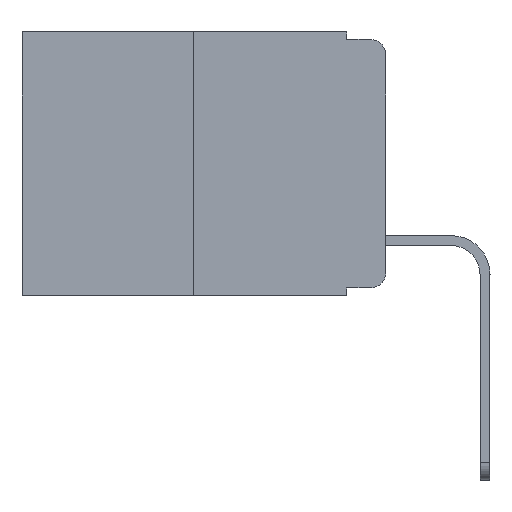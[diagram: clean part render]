
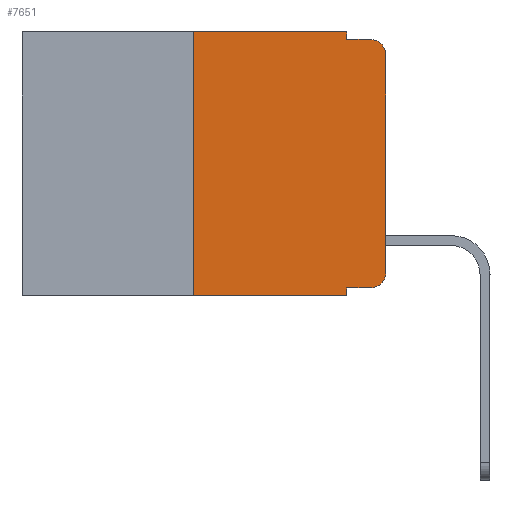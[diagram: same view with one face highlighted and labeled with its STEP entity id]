
A CAD part, left-side view. The second image highlights one B-rep face of the part: STEP entity #7651.
In plain terms, the highlighted planar face has unit normal (-1, 0, 0).
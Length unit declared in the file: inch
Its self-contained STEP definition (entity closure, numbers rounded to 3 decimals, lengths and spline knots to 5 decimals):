
#109 = LINE ( 'NONE', #5461, #2722 ) ;
#172 = ORIENTED_EDGE ( 'NONE', *, *, #11905, .T. ) ;
#251 = EDGE_CURVE ( 'NONE', #7422, #13731, #5358, .T. ) ;
#749 = VERTEX_POINT ( 'NONE', #11626 ) ;
#819 = PLANE ( 'NONE',  #2697 ) ;
#821 = EDGE_CURVE ( 'NONE', #7976, #8249, #10779, .T. ) ;
#843 = EDGE_CURVE ( 'NONE', #11593, #3846, #2901, .T. ) ;
#1059 = EDGE_CURVE ( 'NONE', #8249, #7422, #9546, .T. ) ;
#1072 = CARTESIAN_POINT ( 'NONE',  ( 0., 0.02, -0.01 ) ) ;
#1090 = CARTESIAN_POINT ( 'NONE',  ( 0., 0.051, -0.333 ) ) ;
#1126 = DIRECTION ( 'NONE',  ( 0., -1., 0. ) ) ;
#1204 = VECTOR ( 'NONE', #8884, 39.37008 ) ;
#1284 = EDGE_LOOP ( 'NONE', ( #6960, #8525, #4920, #4372, #13364, #8591, #172, #10805, #10701, #6468 ) ) ;
#1862 = CARTESIAN_POINT ( 'NONE',  ( 0., 0.051, 0. ) ) ;
#1966 = VERTEX_POINT ( 'NONE', #9708 ) ;
#2061 = CARTESIAN_POINT ( 'NONE',  ( 0., 0.25, 0. ) ) ;
#2069 = DIRECTION ( 'NONE',  ( 0., 0., 1. ) ) ;
#2205 = CARTESIAN_POINT ( 'NONE',  ( 0., 0.051, -0.333 ) ) ;
#2697 = AXIS2_PLACEMENT_3D ( 'NONE', #6292, #8699, #10949 ) ;
#2722 = VECTOR ( 'NONE', #2069, 39.37008 ) ;
#2736 = LINE ( 'NONE', #4122, #13785 ) ;
#2757 = VECTOR ( 'NONE', #10697, 39.37008 ) ;
#2901 = CIRCLE ( 'NONE', #11261, 0.02 ) ;
#3228 = EDGE_CURVE ( 'NONE', #12666, #12485, #13107, .T. ) ;
#3245 = CARTESIAN_POINT ( 'NONE',  ( 0., 0.473, -0.343 ) ) ;
#3316 = LINE ( 'NONE', #6410, #9618 ) ;
#3581 = CIRCLE ( 'NONE', #4974, 0.02 ) ;
#3763 = VECTOR ( 'NONE', #1126, 39.37008 ) ;
#3846 = VERTEX_POINT ( 'NONE', #1072 ) ;
#4075 = DIRECTION ( 'NONE',  ( 0., 0., -1. ) ) ;
#4122 = CARTESIAN_POINT ( 'NONE',  ( 0., 0.051, -0.01 ) ) ;
#4372 = ORIENTED_EDGE ( 'NONE', *, *, #251, .F. ) ;
#4920 = ORIENTED_EDGE ( 'NONE', *, *, #11890, .F. ) ;
#4974 = AXIS2_PLACEMENT_3D ( 'NONE', #5979, #13850, #9181 ) ;
#5358 = LINE ( 'NONE', #1862, #2757 ) ;
#5410 = CARTESIAN_POINT ( 'NONE',  ( 0., 0.02, -0.333 ) ) ;
#5430 = DIRECTION ( 'NONE',  ( 0., 0., -1. ) ) ;
#5461 = CARTESIAN_POINT ( 'NONE',  ( 0., 0., 0. ) ) ;
#5529 = DIRECTION ( 'NONE',  ( 0., -1., 0. ) ) ;
#5752 = FACE_OUTER_BOUND ( 'NONE', #1284, .T. ) ;
#5979 = CARTESIAN_POINT ( 'NONE',  ( 0., 0.02, -0.313 ) ) ;
#6290 = CARTESIAN_POINT ( 'NONE',  ( 0., 0.051, -0.01 ) ) ;
#6292 = CARTESIAN_POINT ( 'NONE',  ( 0., 0.473, 0. ) ) ;
#6380 = LINE ( 'NONE', #3245, #14308 ) ;
#6410 = CARTESIAN_POINT ( 'NONE',  ( 0., 0.051, 0. ) ) ;
#6468 = ORIENTED_EDGE ( 'NONE', *, *, #12697, .T. ) ;
#6556 = VECTOR ( 'NONE', #12756, 39.37008 ) ;
#6960 = ORIENTED_EDGE ( 'NONE', *, *, #12525, .T. ) ;
#7189 = CARTESIAN_POINT ( 'NONE',  ( 0., 0.25, 0. ) ) ;
#7422 = VERTEX_POINT ( 'NONE', #8262 ) ;
#7651 = ADVANCED_FACE ( 'NONE', ( #5752 ), #819, .F. ) ;
#7976 = VERTEX_POINT ( 'NONE', #11299 ) ;
#8249 = VERTEX_POINT ( 'NONE', #2061 ) ;
#8262 = CARTESIAN_POINT ( 'NONE',  ( 0., 0.051, 0. ) ) ;
#8525 = ORIENTED_EDGE ( 'NONE', *, *, #843, .T. ) ;
#8591 = ORIENTED_EDGE ( 'NONE', *, *, #821, .F. ) ;
#8616 = DIRECTION ( 'NONE',  ( 0., -1., 0. ) ) ;
#8699 = DIRECTION ( 'NONE',  ( 1., 0., 0. ) ) ;
#8884 = DIRECTION ( 'NONE',  ( 0., -1., 0. ) ) ;
#8893 = EDGE_CURVE ( 'NONE', #12666, #1966, #3316, .T. ) ;
#9181 = DIRECTION ( 'NONE',  ( 0., 0., -1. ) ) ;
#9546 = LINE ( 'NONE', #12134, #3763 ) ;
#9618 = VECTOR ( 'NONE', #5430, 39.37008 ) ;
#9702 = CARTESIAN_POINT ( 'NONE',  ( 0., 0.02, -0.03 ) ) ;
#9708 = CARTESIAN_POINT ( 'NONE',  ( 0., 0.051, -0.343 ) ) ;
#10697 = DIRECTION ( 'NONE',  ( 0., 0., -1. ) ) ;
#10701 = ORIENTED_EDGE ( 'NONE', *, *, #3228, .T. ) ;
#10779 = LINE ( 'NONE', #7189, #6556 ) ;
#10805 = ORIENTED_EDGE ( 'NONE', *, *, #8893, .F. ) ;
#10949 = DIRECTION ( 'NONE',  ( 0., 0., -1. ) ) ;
#11261 = AXIS2_PLACEMENT_3D ( 'NONE', #9702, #14032, #4075 ) ;
#11299 = CARTESIAN_POINT ( 'NONE',  ( 0., 0.25, -0.343 ) ) ;
#11473 = CARTESIAN_POINT ( 'NONE',  ( 0., 0., -0.03 ) ) ;
#11593 = VERTEX_POINT ( 'NONE', #11473 ) ;
#11626 = CARTESIAN_POINT ( 'NONE',  ( 0., 0., -0.313 ) ) ;
#11890 = EDGE_CURVE ( 'NONE', #13731, #3846, #2736, .T. ) ;
#11905 = EDGE_CURVE ( 'NONE', #7976, #1966, #6380, .T. ) ;
#12134 = CARTESIAN_POINT ( 'NONE',  ( 0., 0.473, 0. ) ) ;
#12485 = VERTEX_POINT ( 'NONE', #5410 ) ;
#12525 = EDGE_CURVE ( 'NONE', #749, #11593, #109, .T. ) ;
#12666 = VERTEX_POINT ( 'NONE', #2205 ) ;
#12697 = EDGE_CURVE ( 'NONE', #12485, #749, #3581, .T. ) ;
#12756 = DIRECTION ( 'NONE',  ( 0., 0., 1. ) ) ;
#13107 = LINE ( 'NONE', #1090, #1204 ) ;
#13364 = ORIENTED_EDGE ( 'NONE', *, *, #1059, .F. ) ;
#13731 = VERTEX_POINT ( 'NONE', #6290 ) ;
#13785 = VECTOR ( 'NONE', #8616, 39.37008 ) ;
#13850 = DIRECTION ( 'NONE',  ( -1., 0., 0. ) ) ;
#14032 = DIRECTION ( 'NONE',  ( -1., 0., 0. ) ) ;
#14308 = VECTOR ( 'NONE', #5529, 39.37008 ) ;
